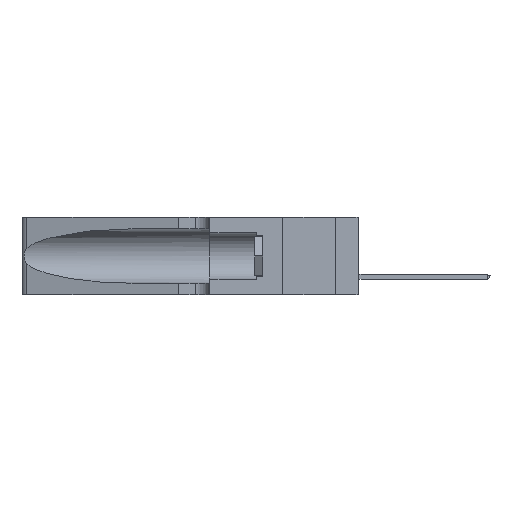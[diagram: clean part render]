
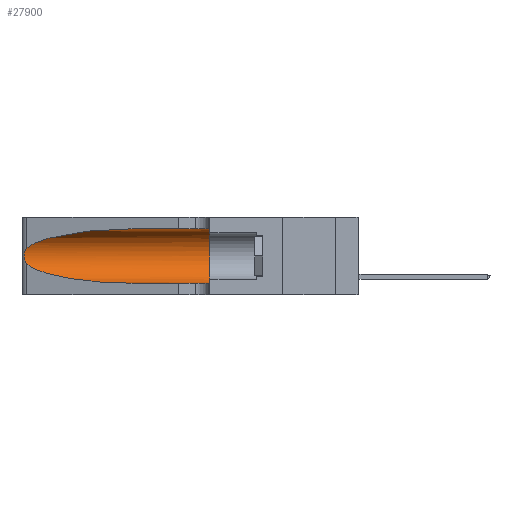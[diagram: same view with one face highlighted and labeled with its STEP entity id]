
A CAD part, left-side view. The second image highlights one B-rep face of the part: STEP entity #27900.
In plain terms, the highlighted cylindrical face has radius 3.308 mm (diameter 6.617 mm), a partial arc.
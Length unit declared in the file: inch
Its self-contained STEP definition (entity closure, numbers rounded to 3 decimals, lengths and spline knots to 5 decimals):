
#978 = VERTEX_POINT ( 'NONE', #25346 ) ;
#1194 = CARTESIAN_POINT ( 'NONE',  ( 0.25639, 1.23186, 0.15144 ) ) ;
#1794 = CARTESIAN_POINT ( 'NONE',  ( 0.26075, 1.23896, 0.19203 ) ) ;
#2402 = EDGE_CURVE ( 'NONE', #36974, #13173, #14439, .T. ) ;
#3342 = VECTOR ( 'NONE', #20432, 39.37008 ) ;
#3797 = B_SPLINE_CURVE_WITH_KNOTS ( 'NONE', 3,
 ( #17967, #37645, #28344, #21527, #12151, #37792, #1794, #34819, #24534, #27771, #11433, #1194, #27189, #17802 ),
 .UNSPECIFIED., .F., .F.,
 ( 4, 2, 2, 2, 2, 2, 4 ),
 ( 0., 0.00027, 0.00053, 0.00107, 0.0016, 0.00187, 0.00214 ),
 .UNSPECIFIED. ) ;
#5025 = CARTESIAN_POINT ( 'NONE',  ( 0.25487, 1.22718, 0.14631 ) ) ;
#5060 = CARTESIAN_POINT ( 'NONE',  ( 0.25487, 1.22718, 0.22369 ) ) ;
#5086 = CARTESIAN_POINT ( 'NONE',  ( 0.1305, 0.72297, 0.05475 ) ) ;
#5334 = DIRECTION ( 'NONE',  ( 0., -1., 0. ) ) ;
#7237 = ORIENTED_EDGE ( 'NONE', *, *, #15998, .T. ) ;
#7378 = CARTESIAN_POINT ( 'NONE',  ( 0.1305, 0.35, 0.31525 ) ) ;
#7505 = CARTESIAN_POINT ( 'NONE',  ( 0.1305, 1.61858, 0.31525 ) ) ;
#8652 = DIRECTION ( 'NONE',  ( 0., 0., 1. ) ) ;
#8812 = ORIENTED_EDGE ( 'NONE', *, *, #33389, .T. ) ;
#9981 = CARTESIAN_POINT ( 'NONE',  ( 0.1305, 1.61858, 0.05475 ) ) ;
#11007 = ORIENTED_EDGE ( 'NONE', *, *, #17491, .T. ) ;
#11433 = CARTESIAN_POINT ( 'NONE',  ( 0.25789, 1.23486, 0.15765 ) ) ;
#11443 = CIRCLE ( 'NONE', #24084, 0.13025 ) ;
#12151 = CARTESIAN_POINT ( 'NONE',  ( 0.25854, 1.2359, 0.20912 ) ) ;
#13173 = VERTEX_POINT ( 'NONE', #28846 ) ;
#13605 = AXIS2_PLACEMENT_3D ( 'NONE', #25392, #5334, #15111 ) ;
#14439 =( BOUNDED_CURVE ( )  B_SPLINE_CURVE ( 3, ( #27641, #24544, #37370, #5060 ),
 .UNSPECIFIED., .F., .F. ) 
 B_SPLINE_CURVE_WITH_KNOTS ( ( 4, 4 ),
 ( 1.5708, 2.84003 ),
 .UNSPECIFIED. ) 
 CURVE ( )  GEOMETRIC_REPRESENTATION_ITEM ( )  RATIONAL_B_SPLINE_CURVE ( ( 1., 0.87, 0.87, 1. ) ) 
 REPRESENTATION_ITEM ( '' )  );
#14689 =( BOUNDED_CURVE ( )  B_SPLINE_CURVE ( 3, ( #36253, #39484, #33573, #20138 ),
 .UNSPECIFIED., .F., .T. ) 
 B_SPLINE_CURVE_WITH_KNOTS ( ( 4, 4 ),
 ( 3.44316, 4.71239 ),
 .UNSPECIFIED. ) 
 CURVE ( )  GEOMETRIC_REPRESENTATION_ITEM ( )  RATIONAL_B_SPLINE_CURVE ( ( 1., 0.87, 0.87, 1. ) ) 
 REPRESENTATION_ITEM ( '' )  );
#15111 = DIRECTION ( 'NONE',  ( 0., 0., -1. ) ) ;
#15621 = DIRECTION ( 'NONE',  ( 0., 1., 0. ) ) ;
#15998 = EDGE_CURVE ( 'NONE', #13173, #16647, #3797, .T. ) ;
#16647 = VERTEX_POINT ( 'NONE', #5025 ) ;
#17491 = EDGE_CURVE ( 'NONE', #16647, #25849, #14689, .T. ) ;
#17802 = CARTESIAN_POINT ( 'NONE',  ( 0.25487, 1.22718, 0.14631 ) ) ;
#17967 = CARTESIAN_POINT ( 'NONE',  ( 0.25487, 1.22718, 0.22369 ) ) ;
#18580 = EDGE_LOOP ( 'NONE', ( #22366, #7237, #11007, #8812, #21551, #38936 ) ) ;
#18615 = CARTESIAN_POINT ( 'NONE',  ( 0.1305, 0.35, 0.185 ) ) ;
#19754 = LINE ( 'NONE', #9981, #27338 ) ;
#19888 = DIRECTION ( 'NONE',  ( 0., -1., 0. ) ) ;
#20138 = CARTESIAN_POINT ( 'NONE',  ( 0.1305, 0.72297, 0.05475 ) ) ;
#20432 = DIRECTION ( 'NONE',  ( 0., -1., 0. ) ) ;
#21527 = CARTESIAN_POINT ( 'NONE',  ( 0.25787, 1.23484, 0.2124 ) ) ;
#21540 = VERTEX_POINT ( 'NONE', #7378 ) ;
#21551 = ORIENTED_EDGE ( 'NONE', *, *, #30095, .F. ) ;
#21815 = CARTESIAN_POINT ( 'NONE',  ( 0.1305, 0.72297, 0.31525 ) ) ;
#22366 = ORIENTED_EDGE ( 'NONE', *, *, #2402, .T. ) ;
#24084 = AXIS2_PLACEMENT_3D ( 'NONE', #18615, #15621, #8652 ) ;
#24534 = CARTESIAN_POINT ( 'NONE',  ( 0.26017, 1.23833, 0.17102 ) ) ;
#24544 = CARTESIAN_POINT ( 'NONE',  ( 0.18966, 0.96281, 0.31525 ) ) ;
#25346 = CARTESIAN_POINT ( 'NONE',  ( 0.1305, 0.35, 0.05475 ) ) ;
#25392 = CARTESIAN_POINT ( 'NONE',  ( 0.1305, 1.61858, 0.185 ) ) ;
#25849 = VERTEX_POINT ( 'NONE', #5086 ) ;
#27189 = CARTESIAN_POINT ( 'NONE',  ( 0.25555, 1.22993, 0.14849 ) ) ;
#27338 = VECTOR ( 'NONE', #19888, 39.37008 ) ;
#27641 = CARTESIAN_POINT ( 'NONE',  ( 0.1305, 0.72297, 0.31525 ) ) ;
#27771 = CARTESIAN_POINT ( 'NONE',  ( 0.25856, 1.23593, 0.16098 ) ) ;
#27861 = FACE_OUTER_BOUND ( 'NONE', #18580, .T. ) ;
#27900 = ADVANCED_FACE ( 'NONE', ( #27861 ), #37955, .F. ) ;
#28344 = CARTESIAN_POINT ( 'NONE',  ( 0.25639, 1.23184, 0.21858 ) ) ;
#28846 = CARTESIAN_POINT ( 'NONE',  ( 0.25487, 1.22718, 0.22369 ) ) ;
#30095 = EDGE_CURVE ( 'NONE', #21540, #978, #11443, .T. ) ;
#33389 = EDGE_CURVE ( 'NONE', #25849, #978, #19754, .T. ) ;
#33573 = CARTESIAN_POINT ( 'NONE',  ( 0.18966, 0.96281, 0.05475 ) ) ;
#34819 = CARTESIAN_POINT ( 'NONE',  ( 0.26075, 1.23896, 0.178 ) ) ;
#36253 = CARTESIAN_POINT ( 'NONE',  ( 0.25487, 1.22718, 0.14631 ) ) ;
#36974 = VERTEX_POINT ( 'NONE', #21815 ) ;
#37370 = CARTESIAN_POINT ( 'NONE',  ( 0.2373, 1.15595, 0.28018 ) ) ;
#37645 = CARTESIAN_POINT ( 'NONE',  ( 0.25555, 1.22994, 0.2215 ) ) ;
#37792 = CARTESIAN_POINT ( 'NONE',  ( 0.26018, 1.23835, 0.19895 ) ) ;
#37955 = CYLINDRICAL_SURFACE ( 'NONE', #13605, 0.13025 ) ;
#38936 = ORIENTED_EDGE ( 'NONE', *, *, #41330, .F. ) ;
#39484 = CARTESIAN_POINT ( 'NONE',  ( 0.2373, 1.15595, 0.08982 ) ) ;
#40826 = LINE ( 'NONE', #7505, #3342 ) ;
#41330 = EDGE_CURVE ( 'NONE', #36974, #21540, #40826, .T. ) ;
